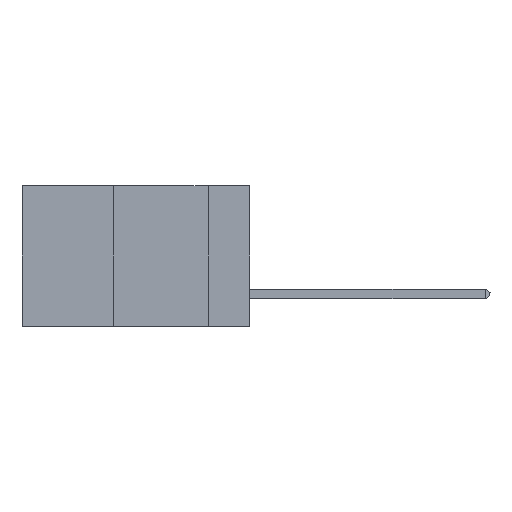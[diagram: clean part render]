
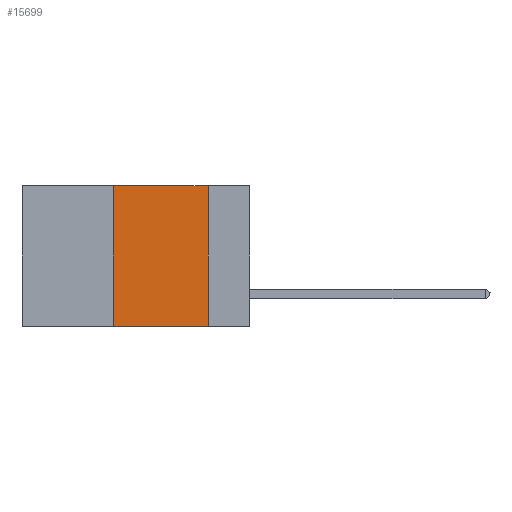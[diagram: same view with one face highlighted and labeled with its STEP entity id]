
A CAD part, left-side view. The second image highlights one B-rep face of the part: STEP entity #15699.
In plain terms, the highlighted planar face has unit normal (-1, 0, 0).
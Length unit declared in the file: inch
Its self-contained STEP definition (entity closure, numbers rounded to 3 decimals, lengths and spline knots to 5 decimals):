
#2354 = LINE ( 'NONE', #11997, #19490 ) ;
#2417 = ORIENTED_EDGE ( 'NONE', *, *, #24080, .F. ) ;
#2717 = LINE ( 'NONE', #16863, #25331 ) ;
#3215 = CARTESIAN_POINT ( 'NONE',  ( 0., 0.6, 0. ) ) ;
#5187 = ORIENTED_EDGE ( 'NONE', *, *, #14201, .F. ) ;
#6925 = EDGE_LOOP ( 'NONE', ( #2417, #5187, #9862, #8744 ) ) ;
#6990 = DIRECTION ( 'NONE',  ( 0., -1., 0. ) ) ;
#7418 = FACE_OUTER_BOUND ( 'NONE', #6925, .T. ) ;
#7709 = CARTESIAN_POINT ( 'NONE',  ( 0., 0.36, -0.37 ) ) ;
#7754 = PLANE ( 'NONE',  #16798 ) ;
#7837 = DIRECTION ( 'NONE',  ( 0., 0., -1. ) ) ;
#8744 = ORIENTED_EDGE ( 'NONE', *, *, #15761, .T. ) ;
#9586 = CARTESIAN_POINT ( 'NONE',  ( 0., 0.11, -0.37 ) ) ;
#9675 = CARTESIAN_POINT ( 'NONE',  ( 0., 0.6, -0.37 ) ) ;
#9759 = DIRECTION ( 'NONE',  ( 1., 0., 0. ) ) ;
#9862 = ORIENTED_EDGE ( 'NONE', *, *, #23612, .F. ) ;
#10166 = CARTESIAN_POINT ( 'NONE',  ( 0., 0.36, 0. ) ) ;
#10307 = LINE ( 'NONE', #9675, #16428 ) ;
#11997 = CARTESIAN_POINT ( 'NONE',  ( 0., 0.11, 0. ) ) ;
#12344 = DIRECTION ( 'NONE',  ( 0., 0., 1. ) ) ;
#12974 = VERTEX_POINT ( 'NONE', #9586 ) ;
#13322 = VERTEX_POINT ( 'NONE', #22018 ) ;
#14024 = VERTEX_POINT ( 'NONE', #10166 ) ;
#14201 = EDGE_CURVE ( 'NONE', #14024, #13322, #18813, .T. ) ;
#14277 = DIRECTION ( 'NONE',  ( 0., 0., -1. ) ) ;
#15699 = ADVANCED_FACE ( 'NONE', ( #7418 ), #7754, .F. ) ;
#15761 = EDGE_CURVE ( 'NONE', #19552, #12974, #10307, .T. ) ;
#16428 = VECTOR ( 'NONE', #24095, 39.37008 ) ;
#16798 = AXIS2_PLACEMENT_3D ( 'NONE', #26269, #9759, #7837 ) ;
#16863 = CARTESIAN_POINT ( 'NONE',  ( 0., 0.36, 0. ) ) ;
#18813 = LINE ( 'NONE', #3215, #25937 ) ;
#19490 = VECTOR ( 'NONE', #14277, 39.37008 ) ;
#19552 = VERTEX_POINT ( 'NONE', #7709 ) ;
#22018 = CARTESIAN_POINT ( 'NONE',  ( 0., 0.11, 0. ) ) ;
#23612 = EDGE_CURVE ( 'NONE', #19552, #14024, #2717, .T. ) ;
#24080 = EDGE_CURVE ( 'NONE', #13322, #12974, #2354, .T. ) ;
#24095 = DIRECTION ( 'NONE',  ( 0., -1., 0. ) ) ;
#25331 = VECTOR ( 'NONE', #12344, 39.37008 ) ;
#25937 = VECTOR ( 'NONE', #6990, 39.37008 ) ;
#26269 = CARTESIAN_POINT ( 'NONE',  ( 0., 0.6, 0. ) ) ;
